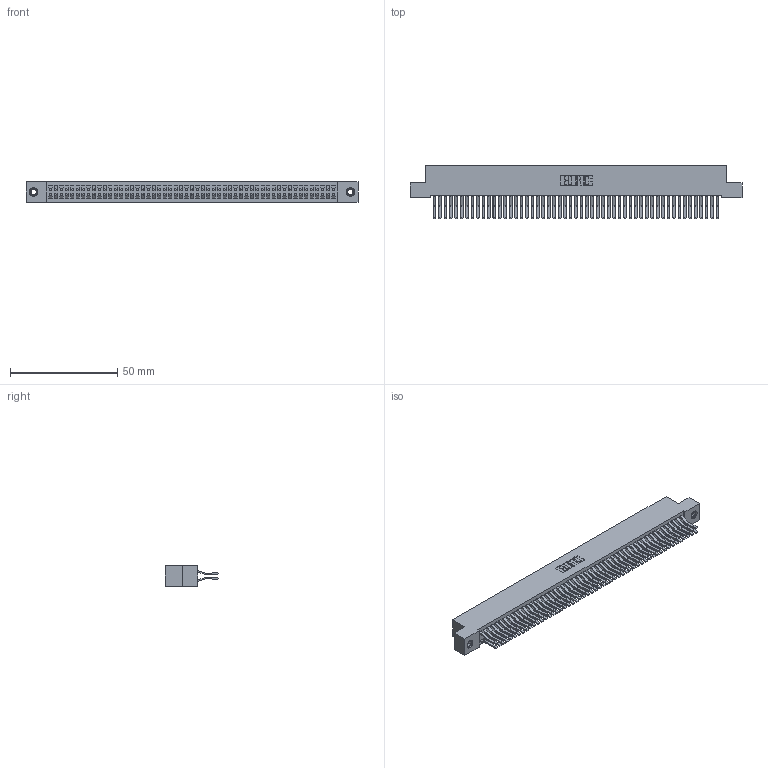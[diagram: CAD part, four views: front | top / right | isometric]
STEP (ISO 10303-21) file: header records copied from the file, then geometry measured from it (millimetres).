
FILE_DESCRIPTION (( 'STEP AP203' ), '1' );
FILE_NAME ('392-106-560-207.STEP', '2019-10-09T22:53:57', ( '' ), ( '' ), 'SwSTEP 2.0', 'SolidWorks 2016', '' );
FILE_SCHEMA (( 'CONFIG_CONTROL_DESIGN' ));
Length unit declared in the file: inch
Products named in the file (4): 342 Part_TI; 345-292-001_560 Tail; 345-250-001_345-250-005-103; 392-106-560-207
Assembly tree (109 placements, depth 2):
  392-106-560-207
    342 Part_TI
    345-292-001_560 Tail  x106
    345-250-001_345-250-005-103  x2
Bounding box: 154.94 x 24.78 x 9.4 mm (x, y, z)
Volume: 14656.6 mm3; surface area: 25822.9 mm2
Topology: 109 solids, 109 shells, 5894 faces, 17501 edges, 11518 vertices
Faces by surface type: plane 3914, cylinder 1964, cone 12, torus 4
Entity records: 33816 total; most frequent: CARTESIAN_POINT 5573, ORIENTED_EDGE 5502, DIRECTION 4777, EDGE_CURVE 2751, VECTOR 2599, LINE 2599, VERTEX_POINT 1828, AXIS2_PLACEMENT_3D 1089
